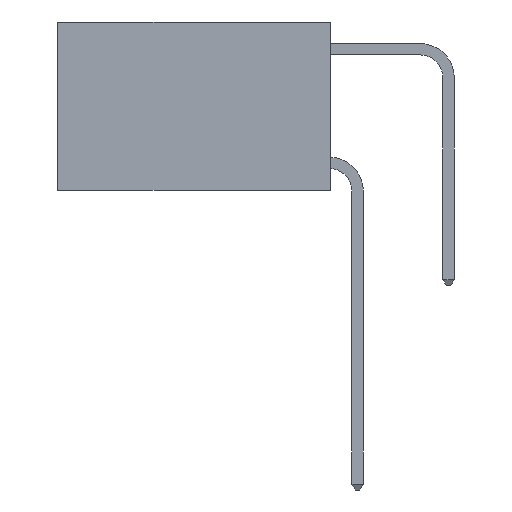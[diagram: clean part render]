
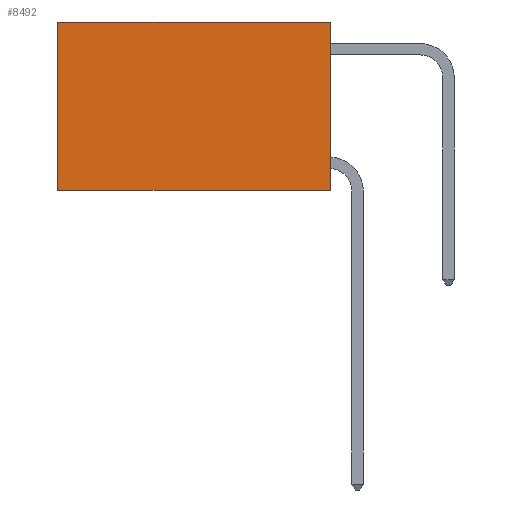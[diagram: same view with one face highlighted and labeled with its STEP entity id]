
A CAD part, left-side view. The second image highlights one B-rep face of the part: STEP entity #8492.
In plain terms, the highlighted planar face has unit normal (-1, 0, 0).
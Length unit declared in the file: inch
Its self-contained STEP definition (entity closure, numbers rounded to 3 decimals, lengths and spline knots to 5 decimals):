
#301 = VERTEX_POINT ( 'NONE', #8559 ) ;
#638 = EDGE_CURVE ( 'NONE', #5043, #1015, #6623, .T. ) ;
#1015 = VERTEX_POINT ( 'NONE', #11680 ) ;
#1248 = LINE ( 'NONE', #11637, #8132 ) ;
#1541 = DIRECTION ( 'NONE',  ( 0., 1., 0. ) ) ;
#1803 = CARTESIAN_POINT ( 'NONE',  ( 0.2625, 0.6, -0.37 ) ) ;
#2706 = LINE ( 'NONE', #7186, #9766 ) ;
#3060 = ORIENTED_EDGE ( 'NONE', *, *, #6697, .F. ) ;
#3322 = EDGE_LOOP ( 'NONE', ( #4184, #3060, #3898, #6463 ) ) ;
#3471 = CARTESIAN_POINT ( 'NONE',  ( 0.2625, 0., 0. ) ) ;
#3898 = ORIENTED_EDGE ( 'NONE', *, *, #11591, .F. ) ;
#4184 = ORIENTED_EDGE ( 'NONE', *, *, #9652, .T. ) ;
#4353 = CARTESIAN_POINT ( 'NONE',  ( 0.2625, 0., 0. ) ) ;
#4403 = CARTESIAN_POINT ( 'NONE',  ( 0.2625, 0., 0. ) ) ;
#4419 = DIRECTION ( 'NONE',  ( 0., 0., -1. ) ) ;
#4433 = DIRECTION ( 'NONE',  ( 1., 0., 0. ) ) ;
#5000 = AXIS2_PLACEMENT_3D ( 'NONE', #3471, #4433, #10808 ) ;
#5043 = VERTEX_POINT ( 'NONE', #4353 ) ;
#5071 = DIRECTION ( 'NONE',  ( 0., 1., 0. ) ) ;
#5247 = DIRECTION ( 'NONE',  ( 0., 0., -1. ) ) ;
#6463 = ORIENTED_EDGE ( 'NONE', *, *, #638, .T. ) ;
#6623 = LINE ( 'NONE', #4403, #11697 ) ;
#6697 = EDGE_CURVE ( 'NONE', #301, #11054, #1248, .T. ) ;
#6777 = VECTOR ( 'NONE', #5247, 39.37008 ) ;
#7186 = CARTESIAN_POINT ( 'NONE',  ( 0.2625, 0., 0. ) ) ;
#7790 = FACE_OUTER_BOUND ( 'NONE', #3322, .T. ) ;
#8072 = CARTESIAN_POINT ( 'NONE',  ( 0.2625, 0.6, 0. ) ) ;
#8132 = VECTOR ( 'NONE', #1541, 39.37008 ) ;
#8492 = ADVANCED_FACE ( 'NONE', ( #7790 ), #9012, .F. ) ;
#8559 = CARTESIAN_POINT ( 'NONE',  ( 0.2625, 0., -0.37 ) ) ;
#9012 = PLANE ( 'NONE',  #5000 ) ;
#9450 = LINE ( 'NONE', #8072, #6777 ) ;
#9652 = EDGE_CURVE ( 'NONE', #1015, #11054, #9450, .T. ) ;
#9766 = VECTOR ( 'NONE', #4419, 39.37008 ) ;
#10808 = DIRECTION ( 'NONE',  ( 0., 0., -1. ) ) ;
#11054 = VERTEX_POINT ( 'NONE', #1803 ) ;
#11591 = EDGE_CURVE ( 'NONE', #5043, #301, #2706, .T. ) ;
#11637 = CARTESIAN_POINT ( 'NONE',  ( 0.2625, 0., -0.37 ) ) ;
#11680 = CARTESIAN_POINT ( 'NONE',  ( 0.2625, 0.6, 0. ) ) ;
#11697 = VECTOR ( 'NONE', #5071, 39.37008 ) ;
